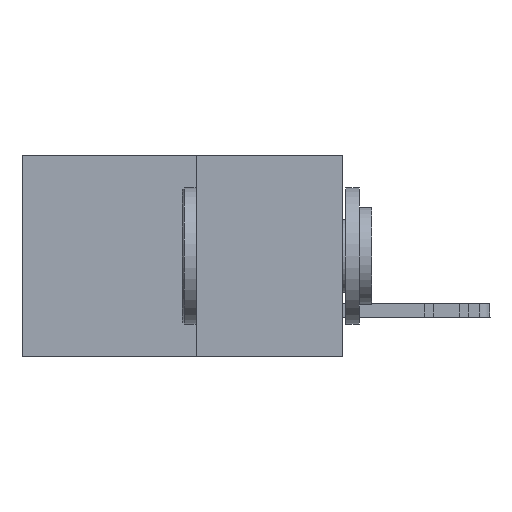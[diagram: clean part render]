
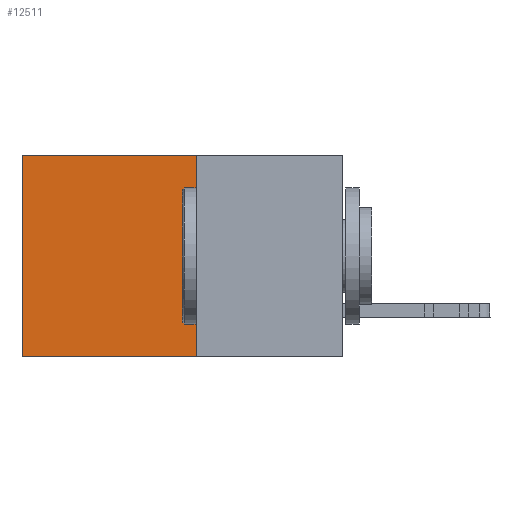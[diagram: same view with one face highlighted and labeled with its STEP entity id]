
A CAD part, left-side view. The second image highlights one B-rep face of the part: STEP entity #12511.
In plain terms, the highlighted planar face has unit normal (-1, 0, 0).
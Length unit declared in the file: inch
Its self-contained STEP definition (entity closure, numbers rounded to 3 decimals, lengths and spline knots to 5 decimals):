
#688 = CARTESIAN_POINT ( 'NONE',  ( 0.277, 0.27, -0.37 ) ) ;
#3870 = VECTOR ( 'NONE', #4770, 39.37008 ) ;
#4343 = AXIS2_PLACEMENT_3D ( 'NONE', #18972, #26837, #11184 ) ;
#4770 = DIRECTION ( 'NONE',  ( 0., 0., -1. ) ) ;
#5586 = DIRECTION ( 'NONE',  ( 0., 1., 0. ) ) ;
#5659 = ORIENTED_EDGE ( 'NONE', *, *, #30142, .T. ) ;
#7899 = VECTOR ( 'NONE', #5586, 39.37008 ) ;
#8151 = VERTEX_POINT ( 'NONE', #27144 ) ;
#8549 = PLANE ( 'NONE',  #4343 ) ;
#8675 = CARTESIAN_POINT ( 'NONE',  ( 0.277, 0.27, 0. ) ) ;
#9389 = VERTEX_POINT ( 'NONE', #8675 ) ;
#10140 = VECTOR ( 'NONE', #15514, 39.37008 ) ;
#10973 = LINE ( 'NONE', #31057, #10140 ) ;
#11184 = DIRECTION ( 'NONE',  ( 0., 0., -1. ) ) ;
#11868 = CARTESIAN_POINT ( 'NONE',  ( 0.277, 0.27, 0. ) ) ;
#12511 = ADVANCED_FACE ( 'NONE', ( #27971 ), #8549, .F. ) ;
#14069 = LINE ( 'NONE', #21253, #7899 ) ;
#15514 = DIRECTION ( 'NONE',  ( 0., 0., -1. ) ) ;
#17089 = ORIENTED_EDGE ( 'NONE', *, *, #27818, .F. ) ;
#17861 = ORIENTED_EDGE ( 'NONE', *, *, #33630, .F. ) ;
#18197 = LINE ( 'NONE', #11868, #32004 ) ;
#18972 = CARTESIAN_POINT ( 'NONE',  ( 0.277, 0.27, -0.37 ) ) ;
#19420 = ORIENTED_EDGE ( 'NONE', *, *, #21084, .T. ) ;
#19635 = DIRECTION ( 'NONE',  ( 0., 1., 0. ) ) ;
#21084 = EDGE_CURVE ( 'NONE', #9389, #8151, #18197, .T. ) ;
#21253 = CARTESIAN_POINT ( 'NONE',  ( 0.277, 0.27, -0.37 ) ) ;
#22880 = VERTEX_POINT ( 'NONE', #26679 ) ;
#23100 = CARTESIAN_POINT ( 'NONE',  ( 0.277, 0.59, -0.37 ) ) ;
#23846 = EDGE_LOOP ( 'NONE', ( #5659, #17861, #17089, #19420 ) ) ;
#26168 = VERTEX_POINT ( 'NONE', #688 ) ;
#26679 = CARTESIAN_POINT ( 'NONE',  ( 0.277, 0.59, -0.37 ) ) ;
#26837 = DIRECTION ( 'NONE',  ( 1., 0., 0. ) ) ;
#27144 = CARTESIAN_POINT ( 'NONE',  ( 0.277, 0.59, 0. ) ) ;
#27818 = EDGE_CURVE ( 'NONE', #9389, #26168, #10973, .T. ) ;
#27971 = FACE_OUTER_BOUND ( 'NONE', #23846, .T. ) ;
#30142 = EDGE_CURVE ( 'NONE', #8151, #22880, #30819, .T. ) ;
#30819 = LINE ( 'NONE', #23100, #3870 ) ;
#31057 = CARTESIAN_POINT ( 'NONE',  ( 0.277, 0.27, -0.37 ) ) ;
#32004 = VECTOR ( 'NONE', #19635, 39.37008 ) ;
#33630 = EDGE_CURVE ( 'NONE', #26168, #22880, #14069, .T. ) ;
